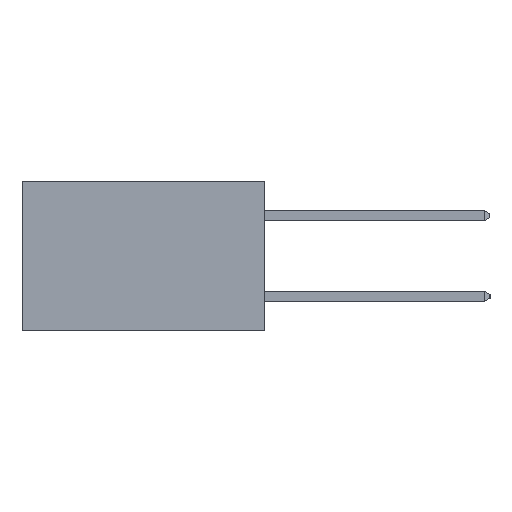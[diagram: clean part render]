
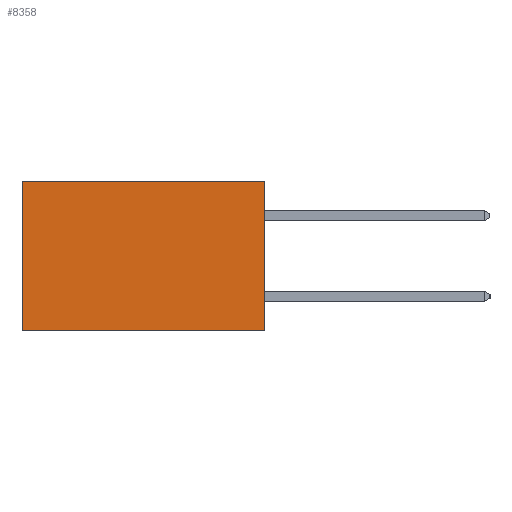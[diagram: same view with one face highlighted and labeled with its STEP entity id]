
A CAD part, left-side view. The second image highlights one B-rep face of the part: STEP entity #8358.
In plain terms, the highlighted planar face has unit normal (-1, 0, 0).
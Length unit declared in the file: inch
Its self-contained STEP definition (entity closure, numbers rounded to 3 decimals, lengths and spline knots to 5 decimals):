
#99 = CARTESIAN_POINT ( 'NONE',  ( 0.2615, 0., 0. ) ) ;
#208 = VERTEX_POINT ( 'NONE', #6819 ) ;
#217 = VECTOR ( 'NONE', #709, 39.37008 ) ;
#406 = VERTEX_POINT ( 'NONE', #5098 ) ;
#649 = DIRECTION ( 'NONE',  ( 0., 0., -1. ) ) ;
#656 = EDGE_CURVE ( 'NONE', #10505, #208, #7649, .T. ) ;
#709 = DIRECTION ( 'NONE',  ( 0., 0., -1. ) ) ;
#735 = CARTESIAN_POINT ( 'NONE',  ( 0.2615, 0.6, -0.37 ) ) ;
#1429 = DIRECTION ( 'NONE',  ( 0., 1., 0. ) ) ;
#1441 = AXIS2_PLACEMENT_3D ( 'NONE', #6012, #5878, #5798 ) ;
#1522 = ORIENTED_EDGE ( 'NONE', *, *, #10353, .T. ) ;
#1850 = CARTESIAN_POINT ( 'NONE',  ( 0.2615, 0., -0.37 ) ) ;
#2184 = EDGE_LOOP ( 'NONE', ( #1522, #5292, #2556, #5897 ) ) ;
#2556 = ORIENTED_EDGE ( 'NONE', *, *, #656, .F. ) ;
#3082 = LINE ( 'NONE', #1850, #5216 ) ;
#4790 = FACE_OUTER_BOUND ( 'NONE', #2184, .T. ) ;
#5098 = CARTESIAN_POINT ( 'NONE',  ( 0.2615, 0.6, 0. ) ) ;
#5175 = VECTOR ( 'NONE', #649, 39.37008 ) ;
#5216 = VECTOR ( 'NONE', #1429, 39.37008 ) ;
#5292 = ORIENTED_EDGE ( 'NONE', *, *, #9014, .F. ) ;
#5517 = EDGE_CURVE ( 'NONE', #10505, #406, #8933, .T. ) ;
#5798 = DIRECTION ( 'NONE',  ( 0., 0., -1. ) ) ;
#5878 = DIRECTION ( 'NONE',  ( 1., 0., 0. ) ) ;
#5897 = ORIENTED_EDGE ( 'NONE', *, *, #5517, .T. ) ;
#5997 = PLANE ( 'NONE',  #1441 ) ;
#6012 = CARTESIAN_POINT ( 'NONE',  ( 0.2615, 0., -0.37 ) ) ;
#6160 = VECTOR ( 'NONE', #6592, 39.37008 ) ;
#6469 = CARTESIAN_POINT ( 'NONE',  ( 0.2615, 0., 0. ) ) ;
#6592 = DIRECTION ( 'NONE',  ( 0., 1., 0. ) ) ;
#6819 = CARTESIAN_POINT ( 'NONE',  ( 0.2615, 0., -0.37 ) ) ;
#7381 = LINE ( 'NONE', #735, #217 ) ;
#7649 = LINE ( 'NONE', #11496, #5175 ) ;
#7654 = CARTESIAN_POINT ( 'NONE',  ( 0.2615, 0.6, -0.37 ) ) ;
#8358 = ADVANCED_FACE ( 'NONE', ( #4790 ), #5997, .F. ) ;
#8933 = LINE ( 'NONE', #6469, #6160 ) ;
#9014 = EDGE_CURVE ( 'NONE', #208, #11840, #3082, .T. ) ;
#10353 = EDGE_CURVE ( 'NONE', #406, #11840, #7381, .T. ) ;
#10505 = VERTEX_POINT ( 'NONE', #99 ) ;
#11496 = CARTESIAN_POINT ( 'NONE',  ( 0.2615, 0., -0.37 ) ) ;
#11840 = VERTEX_POINT ( 'NONE', #7654 ) ;
